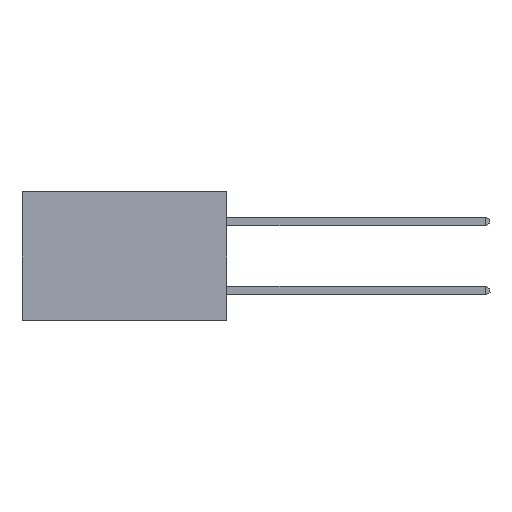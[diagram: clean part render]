
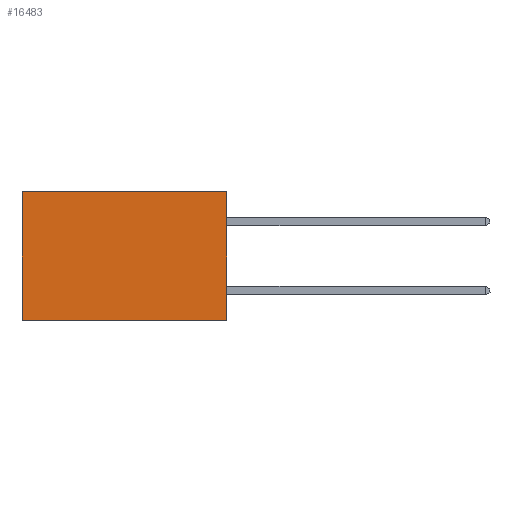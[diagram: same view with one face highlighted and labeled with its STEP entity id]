
A CAD part, left-side view. The second image highlights one B-rep face of the part: STEP entity #16483.
In plain terms, the highlighted planar face has unit normal (-1, 0, 0).
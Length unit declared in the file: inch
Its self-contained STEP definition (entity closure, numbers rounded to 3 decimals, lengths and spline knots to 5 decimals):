
#339 = VECTOR ( 'NONE', #13786, 39.37008 ) ;
#1142 = FACE_OUTER_BOUND ( 'NONE', #9192, .T. ) ;
#1333 = EDGE_CURVE ( 'NONE', #12678, #28142, #15209, .T. ) ;
#2018 = DIRECTION ( 'NONE',  ( 0., 0., -1. ) ) ;
#2908 = CARTESIAN_POINT ( 'NONE',  ( 0.277, 0., -0.37 ) ) ;
#4687 = EDGE_CURVE ( 'NONE', #12678, #16681, #20386, .T. ) ;
#8209 = ORIENTED_EDGE ( 'NONE', *, *, #1333, .F. ) ;
#9192 = EDGE_LOOP ( 'NONE', ( #20256, #23927, #8209, #13535 ) ) ;
#9648 = AXIS2_PLACEMENT_3D ( 'NONE', #17693, #15593, #2018 ) ;
#9839 = CARTESIAN_POINT ( 'NONE',  ( 0.277, 0., -0.37 ) ) ;
#9983 = VECTOR ( 'NONE', #28237, 39.37008 ) ;
#11119 = EDGE_CURVE ( 'NONE', #16681, #17028, #13873, .T. ) ;
#12678 = VERTEX_POINT ( 'NONE', #28693 ) ;
#13354 = PLANE ( 'NONE',  #9648 ) ;
#13535 = ORIENTED_EDGE ( 'NONE', *, *, #4687, .T. ) ;
#13683 = CARTESIAN_POINT ( 'NONE',  ( 0.277, 0.59, -0.37 ) ) ;
#13786 = DIRECTION ( 'NONE',  ( 0., 0., -1. ) ) ;
#13873 = LINE ( 'NONE', #13683, #339 ) ;
#15209 = LINE ( 'NONE', #2908, #26287 ) ;
#15593 = DIRECTION ( 'NONE',  ( 1., 0., 0. ) ) ;
#16483 = ADVANCED_FACE ( 'NONE', ( #1142 ), #13354, .F. ) ;
#16681 = VERTEX_POINT ( 'NONE', #24968 ) ;
#17028 = VERTEX_POINT ( 'NONE', #23902 ) ;
#17693 = CARTESIAN_POINT ( 'NONE',  ( 0.277, 0., -0.37 ) ) ;
#18853 = VECTOR ( 'NONE', #23008, 39.37008 ) ;
#19355 = DIRECTION ( 'NONE',  ( 0., 0., -1. ) ) ;
#20256 = ORIENTED_EDGE ( 'NONE', *, *, #11119, .T. ) ;
#20386 = LINE ( 'NONE', #28295, #9983 ) ;
#20782 = CARTESIAN_POINT ( 'NONE',  ( 0.277, 0., -0.37 ) ) ;
#23008 = DIRECTION ( 'NONE',  ( 0., 1., 0. ) ) ;
#23416 = EDGE_CURVE ( 'NONE', #28142, #17028, #24745, .T. ) ;
#23902 = CARTESIAN_POINT ( 'NONE',  ( 0.277, 0.59, -0.37 ) ) ;
#23927 = ORIENTED_EDGE ( 'NONE', *, *, #23416, .F. ) ;
#24745 = LINE ( 'NONE', #20782, #18853 ) ;
#24968 = CARTESIAN_POINT ( 'NONE',  ( 0.277, 0.59, 0. ) ) ;
#26287 = VECTOR ( 'NONE', #19355, 39.37008 ) ;
#28142 = VERTEX_POINT ( 'NONE', #9839 ) ;
#28237 = DIRECTION ( 'NONE',  ( 0., 1., 0. ) ) ;
#28295 = CARTESIAN_POINT ( 'NONE',  ( 0.277, 0., 0. ) ) ;
#28693 = CARTESIAN_POINT ( 'NONE',  ( 0.277, 0., 0. ) ) ;
